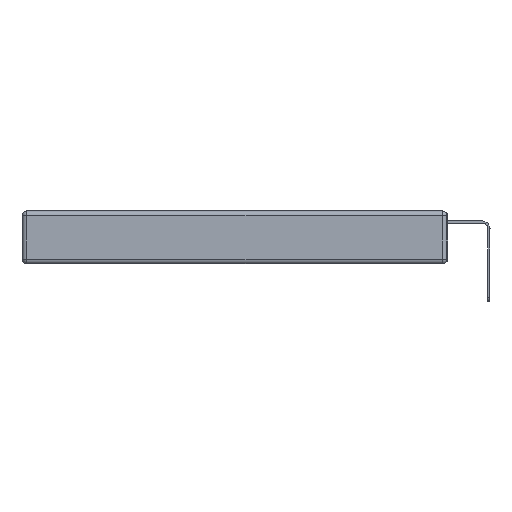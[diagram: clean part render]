
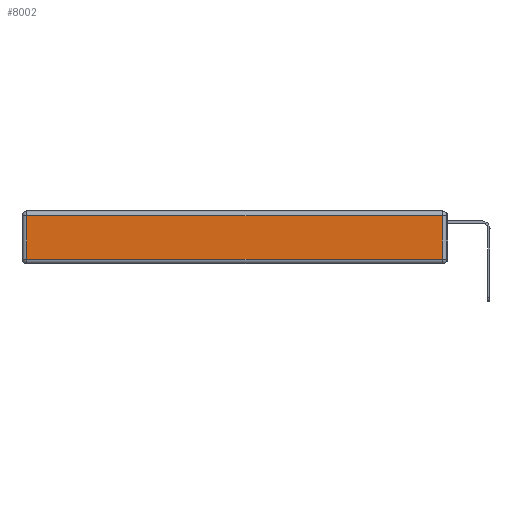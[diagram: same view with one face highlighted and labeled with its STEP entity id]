
A CAD part, left-side view. The second image highlights one B-rep face of the part: STEP entity #8002.
In plain terms, the highlighted planar face has unit normal (-1, 0, 0).
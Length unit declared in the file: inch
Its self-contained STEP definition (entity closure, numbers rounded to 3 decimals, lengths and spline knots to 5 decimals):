
#392 = VERTEX_POINT ( 'NONE', #12229 ) ;
#1406 = LINE ( 'NONE', #11802, #2321 ) ;
#1820 = CARTESIAN_POINT ( 'NONE',  ( 0., 0.03, -0.343 ) ) ;
#2321 = VECTOR ( 'NONE', #17554, 39.37008 ) ;
#2814 = VECTOR ( 'NONE', #19305, 39.37008 ) ;
#3230 = CARTESIAN_POINT ( 'NONE',  ( 0., 0.03, -0.03 ) ) ;
#4904 = LINE ( 'NONE', #22923, #2814 ) ;
#5547 = PLANE ( 'NONE',  #24475 ) ;
#5913 = VERTEX_POINT ( 'NONE', #3230 ) ;
#5953 = VECTOR ( 'NONE', #6993, 39.37008 ) ;
#6993 = DIRECTION ( 'NONE',  ( 0., 1., 0. ) ) ;
#8002 = ADVANCED_FACE ( 'NONE', ( #22523 ), #5547, .T. ) ;
#8082 = DIRECTION ( 'NONE',  ( 0., 0., 1. ) ) ;
#8233 = VECTOR ( 'NONE', #15268, 39.37008 ) ;
#8297 = EDGE_CURVE ( 'NONE', #5913, #392, #19813, .T. ) ;
#8850 = LINE ( 'NONE', #1820, #8233 ) ;
#10840 = CARTESIAN_POINT ( 'NONE',  ( 0., 2.72, -0.313 ) ) ;
#11802 = CARTESIAN_POINT ( 'NONE',  ( 0., 2.72, -0.343 ) ) ;
#12229 = CARTESIAN_POINT ( 'NONE',  ( 0., 2.72, -0.03 ) ) ;
#13808 = EDGE_CURVE ( 'NONE', #392, #17173, #1406, .T. ) ;
#14436 = ORIENTED_EDGE ( 'NONE', *, *, #20735, .T. ) ;
#14864 = ORIENTED_EDGE ( 'NONE', *, *, #8297, .T. ) ;
#14896 = ORIENTED_EDGE ( 'NONE', *, *, #20780, .T. ) ;
#15193 = ORIENTED_EDGE ( 'NONE', *, *, #13808, .T. ) ;
#15268 = DIRECTION ( 'NONE',  ( 0., 0., 1. ) ) ;
#17173 = VERTEX_POINT ( 'NONE', #10840 ) ;
#17554 = DIRECTION ( 'NONE',  ( 0., 0., -1. ) ) ;
#19305 = DIRECTION ( 'NONE',  ( 0., -1., 0. ) ) ;
#19583 = DIRECTION ( 'NONE',  ( -1., 0., 0. ) ) ;
#19813 = LINE ( 'NONE', #20343, #5953 ) ;
#20343 = CARTESIAN_POINT ( 'NONE',  ( 0., 2.75, -0.03 ) ) ;
#20369 = VERTEX_POINT ( 'NONE', #21767 ) ;
#20735 = EDGE_CURVE ( 'NONE', #17173, #20369, #4904, .T. ) ;
#20780 = EDGE_CURVE ( 'NONE', #20369, #5913, #8850, .T. ) ;
#21003 = CARTESIAN_POINT ( 'NONE',  ( 0., 0., -0.343 ) ) ;
#21767 = CARTESIAN_POINT ( 'NONE',  ( 0., 0.03, -0.313 ) ) ;
#21960 = EDGE_LOOP ( 'NONE', ( #14436, #14896, #14864, #15193 ) ) ;
#22523 = FACE_OUTER_BOUND ( 'NONE', #21960, .T. ) ;
#22923 = CARTESIAN_POINT ( 'NONE',  ( 0., 0., -0.313 ) ) ;
#24475 = AXIS2_PLACEMENT_3D ( 'NONE', #21003, #19583, #8082 ) ;
